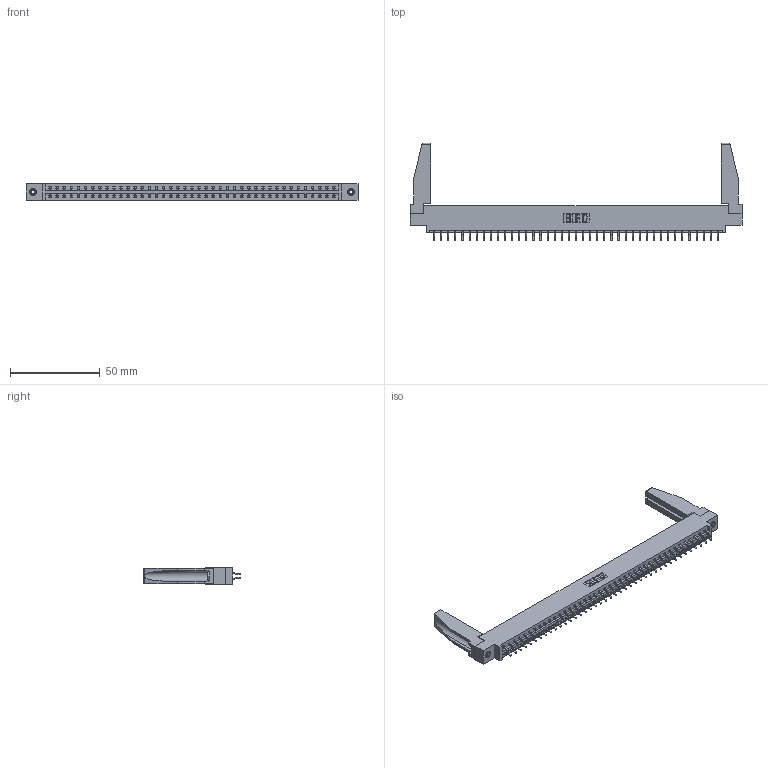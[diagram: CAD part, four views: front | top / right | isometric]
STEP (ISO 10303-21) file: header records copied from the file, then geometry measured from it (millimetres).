
FILE_DESCRIPTION (( 'STEP AP203' ), '1' );
FILE_NAME ('337-082-556-878.STEP', '2019-10-15T17:31:27', ( '' ), ( '' ), 'SwSTEP 2.0', 'SolidWorks 2016', '' );
FILE_SCHEMA (( 'CONFIG_CONTROL_DESIGN' ));
Length unit declared in the file: inch
Products named in the file (5): 307-220-078; 345-250-001_345-250-001-102; 345-292-001_556 Tail; 337 Part_0.170 Offset - 0.156 Dia-TI; 337-082-556-878
Assembly tree (87 placements, depth 2):
  337-082-556-878
    337 Part_0.170 Offset - 0.156 Dia-TI
    345-292-001_556 Tail  x82
    345-250-001_345-250-001-102  x2
    307-220-078  x2
Bounding box: 185.47 x 54.37 x 9.4 mm (x, y, z)
Volume: 23405.7 mm3; surface area: 25787.7 mm2
Topology: 87 solids, 87 shells, 5168 faces, 15331 edges, 10102 vertices
Faces by surface type: plane 3602, cylinder 1550, cone 12, torus 4
Entity records: 34710 total; most frequent: CARTESIAN_POINT 5864, ORIENTED_EDGE 5744, DIRECTION 4984, EDGE_CURVE 2872, LINE 2698, VECTOR 2698, VERTEX_POINT 1908, AXIS2_PLACEMENT_3D 1143
